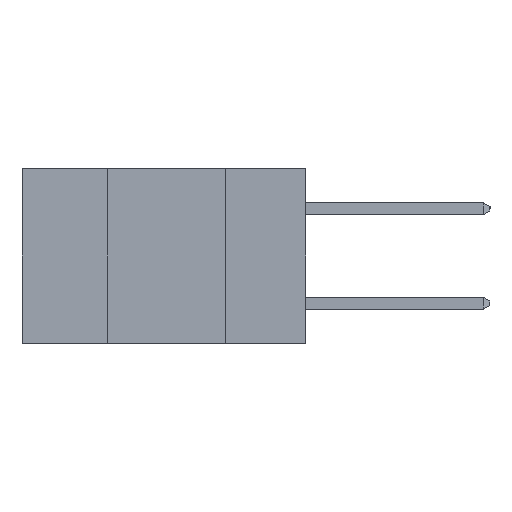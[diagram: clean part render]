
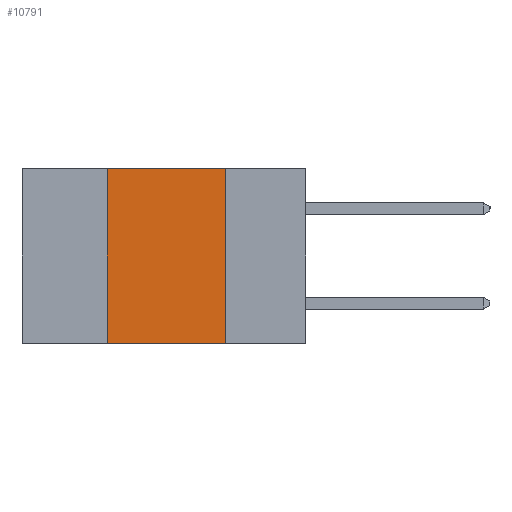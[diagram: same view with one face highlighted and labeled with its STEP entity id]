
A CAD part, left-side view. The second image highlights one B-rep face of the part: STEP entity #10791.
In plain terms, the highlighted planar face has unit normal (-1, 0, 0).
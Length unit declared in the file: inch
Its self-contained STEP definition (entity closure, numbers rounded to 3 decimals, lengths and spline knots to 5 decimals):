
#891 = DIRECTION ( 'NONE',  ( 0., -1., 0. ) ) ;
#1860 = AXIS2_PLACEMENT_3D ( 'NONE', #11556, #7998, #12734 ) ;
#1929 = EDGE_CURVE ( 'NONE', #15172, #10309, #12653, .T. ) ;
#3222 = FACE_OUTER_BOUND ( 'NONE', #13975, .T. ) ;
#3371 = VERTEX_POINT ( 'NONE', #5179 ) ;
#3464 = CARTESIAN_POINT ( 'NONE',  ( 0., 0.17, 0. ) ) ;
#3603 = LINE ( 'NONE', #4996, #12058 ) ;
#4241 = EDGE_CURVE ( 'NONE', #3371, #13895, #10810, .T. ) ;
#4672 = VECTOR ( 'NONE', #12879, 39.37008 ) ;
#4996 = CARTESIAN_POINT ( 'NONE',  ( 0., 0.42, -0.37 ) ) ;
#5179 = CARTESIAN_POINT ( 'NONE',  ( 0., 0.42, 0. ) ) ;
#5660 = DIRECTION ( 'NONE',  ( 0., 0., -1. ) ) ;
#5832 = CARTESIAN_POINT ( 'NONE',  ( 0., 0.6, 0. ) ) ;
#7998 = DIRECTION ( 'NONE',  ( 1., 0., 0. ) ) ;
#8209 = CARTESIAN_POINT ( 'NONE',  ( 0., 0.6, -0.37 ) ) ;
#8375 = ORIENTED_EDGE ( 'NONE', *, *, #1929, .T. ) ;
#9773 = DIRECTION ( 'NONE',  ( 0., 0., 1. ) ) ;
#10309 = VERTEX_POINT ( 'NONE', #11722 ) ;
#10672 = ORIENTED_EDGE ( 'NONE', *, *, #4241, .F. ) ;
#10791 = ADVANCED_FACE ( 'NONE', ( #3222 ), #13825, .F. ) ;
#10810 = LINE ( 'NONE', #5832, #4672 ) ;
#11355 = LINE ( 'NONE', #11504, #12097 ) ;
#11504 = CARTESIAN_POINT ( 'NONE',  ( 0., 0.17, -0.37 ) ) ;
#11556 = CARTESIAN_POINT ( 'NONE',  ( 0., 0.6, 0. ) ) ;
#11651 = ORIENTED_EDGE ( 'NONE', *, *, #12063, .F. ) ;
#11722 = CARTESIAN_POINT ( 'NONE',  ( 0., 0.17, -0.37 ) ) ;
#12058 = VECTOR ( 'NONE', #9773, 39.37008 ) ;
#12063 = EDGE_CURVE ( 'NONE', #15172, #3371, #3603, .T. ) ;
#12097 = VECTOR ( 'NONE', #5660, 39.37008 ) ;
#12653 = LINE ( 'NONE', #8209, #13658 ) ;
#12734 = DIRECTION ( 'NONE',  ( 0., 0., -1. ) ) ;
#12879 = DIRECTION ( 'NONE',  ( 0., -1., 0. ) ) ;
#12991 = CARTESIAN_POINT ( 'NONE',  ( 0., 0.42, -0.37 ) ) ;
#13658 = VECTOR ( 'NONE', #891, 39.37008 ) ;
#13800 = EDGE_CURVE ( 'NONE', #13895, #10309, #11355, .T. ) ;
#13825 = PLANE ( 'NONE',  #1860 ) ;
#13895 = VERTEX_POINT ( 'NONE', #3464 ) ;
#13975 = EDGE_LOOP ( 'NONE', ( #15215, #10672, #11651, #8375 ) ) ;
#15172 = VERTEX_POINT ( 'NONE', #12991 ) ;
#15215 = ORIENTED_EDGE ( 'NONE', *, *, #13800, .F. ) ;
